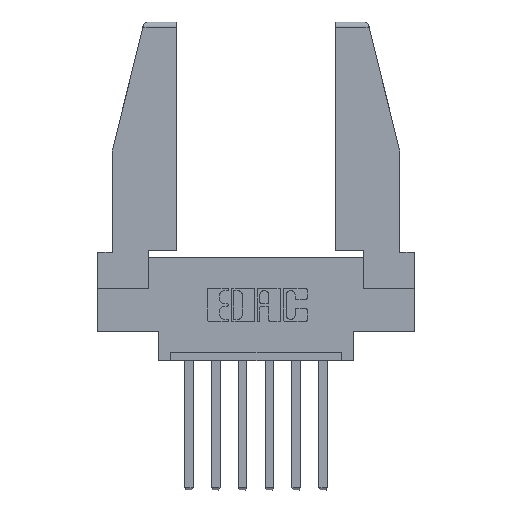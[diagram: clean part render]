
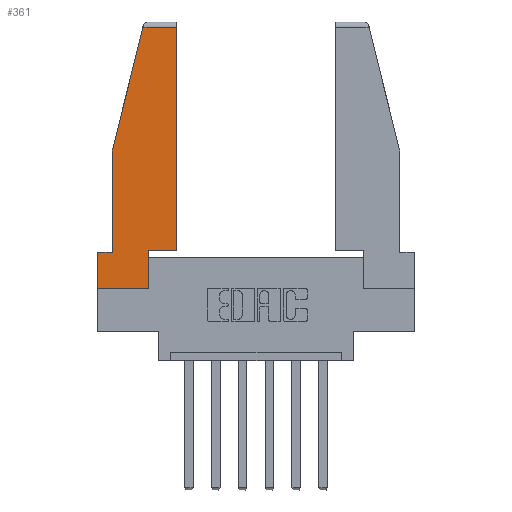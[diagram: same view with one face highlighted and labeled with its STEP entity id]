
A CAD part, top view. The second image highlights one B-rep face of the part: STEP entity #361.
In plain terms, the highlighted planar face has unit normal (0, 0, 1).
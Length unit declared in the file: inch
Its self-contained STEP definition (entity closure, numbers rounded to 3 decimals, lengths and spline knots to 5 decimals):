
#76 = VECTOR ( 'NONE', #7439, 39.37008 ) ;
#149 = VECTOR ( 'NONE', #5746, 39.37008 ) ;
#361 = ADVANCED_FACE ( 'NONE', ( #3894 ), #3486, .T. ) ;
#385 = CARTESIAN_POINT ( 'NONE',  ( 0., 0.21, 0. ) ) ;
#626 = ORIENTED_EDGE ( 'NONE', *, *, #6270, .T. ) ;
#740 = EDGE_CURVE ( 'NONE', #3616, #10870, #2608, .T. ) ;
#2084 = VECTOR ( 'NONE', #3335, 39.37008 ) ;
#2313 = LINE ( 'NONE', #10133, #11498 ) ;
#2318 = ORIENTED_EDGE ( 'NONE', *, *, #4120, .T. ) ;
#2553 = VERTEX_POINT ( 'NONE', #7074 ) ;
#2608 = LINE ( 'NONE', #7267, #2751 ) ;
#2626 = VECTOR ( 'NONE', #10474, 39.37008 ) ;
#2751 = VECTOR ( 'NONE', #9202, 39.37008 ) ;
#3041 = CARTESIAN_POINT ( 'NONE',  ( 0.086, 0.21, 0. ) ) ;
#3116 = ORIENTED_EDGE ( 'NONE', *, *, #9472, .T. ) ;
#3146 = CARTESIAN_POINT ( 'NONE',  ( 0.2636, 1.52, 0. ) ) ;
#3170 = VECTOR ( 'NONE', #8428, 39.37008 ) ;
#3335 = DIRECTION ( 'NONE',  ( 0., -1., 0. ) ) ;
#3486 = PLANE ( 'NONE',  #11102 ) ;
#3616 = VERTEX_POINT ( 'NONE', #3146 ) ;
#3618 = LINE ( 'NONE', #9790, #2626 ) ;
#3780 = LINE ( 'NONE', #10277, #149 ) ;
#3782 = ORIENTED_EDGE ( 'NONE', *, *, #4172, .T. ) ;
#3845 = DIRECTION ( 'NONE',  ( 1., 0., 0. ) ) ;
#3894 = FACE_OUTER_BOUND ( 'NONE', #5212, .T. ) ;
#4120 = EDGE_CURVE ( 'NONE', #10870, #5507, #9185, .T. ) ;
#4172 = EDGE_CURVE ( 'NONE', #7323, #3616, #5680, .T. ) ;
#4372 = DIRECTION ( 'NONE',  ( 1., 0., 0. ) ) ;
#4837 = CARTESIAN_POINT ( 'NONE',  ( 0.086, 0.8, 0. ) ) ;
#5212 = EDGE_LOOP ( 'NONE', ( #7995, #3782, #9319, #2318, #3116, #6295, #626, #8586, #10837 ) ) ;
#5507 = VERTEX_POINT ( 'NONE', #3041 ) ;
#5680 = LINE ( 'NONE', #6605, #3170 ) ;
#5708 = CARTESIAN_POINT ( 'NONE',  ( 0.297, 0.223, 0. ) ) ;
#5746 = DIRECTION ( 'NONE',  ( 0., 1., 0. ) ) ;
#5966 = VECTOR ( 'NONE', #7519, 39.37008 ) ;
#6060 = VECTOR ( 'NONE', #10215, 39.37008 ) ;
#6270 = EDGE_CURVE ( 'NONE', #10476, #2553, #2313, .T. ) ;
#6295 = ORIENTED_EDGE ( 'NONE', *, *, #9051, .T. ) ;
#6425 = EDGE_CURVE ( 'NONE', #9236, #7323, #8443, .T. ) ;
#6564 = EDGE_CURVE ( 'NONE', #10637, #9236, #10944, .T. ) ;
#6605 = CARTESIAN_POINT ( 'NONE',  ( 0., 1.52, 0. ) ) ;
#6821 = CARTESIAN_POINT ( 'NONE',  ( 0.461, 1.52, 0. ) ) ;
#7074 = CARTESIAN_POINT ( 'NONE',  ( 0.297, 0., 0. ) ) ;
#7140 = CARTESIAN_POINT ( 'NONE',  ( 0., 0., 0. ) ) ;
#7267 = CARTESIAN_POINT ( 'NONE',  ( 0.271, 1.55, 0. ) ) ;
#7323 = VERTEX_POINT ( 'NONE', #6821 ) ;
#7439 = DIRECTION ( 'NONE',  ( 1., 0., 0. ) ) ;
#7519 = DIRECTION ( 'NONE',  ( 0., -1., 0. ) ) ;
#7605 = CARTESIAN_POINT ( 'NONE',  ( 0.086, 0.8, 0. ) ) ;
#7822 = LINE ( 'NONE', #10575, #2084 ) ;
#7995 = ORIENTED_EDGE ( 'NONE', *, *, #6425, .T. ) ;
#8428 = DIRECTION ( 'NONE',  ( -1., 0., 0. ) ) ;
#8443 = LINE ( 'NONE', #8508, #6060 ) ;
#8455 = CARTESIAN_POINT ( 'NONE',  ( 0.297, 0.223, 0. ) ) ;
#8507 = CARTESIAN_POINT ( 'NONE',  ( 0., 0., 0. ) ) ;
#8508 = CARTESIAN_POINT ( 'NONE',  ( 0.461, 0.223, 0. ) ) ;
#8586 = ORIENTED_EDGE ( 'NONE', *, *, #8911, .T. ) ;
#8911 = EDGE_CURVE ( 'NONE', #2553, #10637, #3780, .T. ) ;
#8949 = DIRECTION ( 'NONE',  ( 0., 0., 1. ) ) ;
#9021 = CARTESIAN_POINT ( 'NONE',  ( 0.461, 0.223, 0. ) ) ;
#9051 = EDGE_CURVE ( 'NONE', #9625, #10476, #7822, .T. ) ;
#9185 = LINE ( 'NONE', #7605, #5966 ) ;
#9202 = DIRECTION ( 'NONE',  ( -0.239, -0.971, 0. ) ) ;
#9236 = VERTEX_POINT ( 'NONE', #9021 ) ;
#9319 = ORIENTED_EDGE ( 'NONE', *, *, #740, .T. ) ;
#9472 = EDGE_CURVE ( 'NONE', #5507, #9625, #3618, .T. ) ;
#9625 = VERTEX_POINT ( 'NONE', #385 ) ;
#9790 = CARTESIAN_POINT ( 'NONE',  ( 0., 0.21, 0. ) ) ;
#10133 = CARTESIAN_POINT ( 'NONE',  ( 0., 0., 0. ) ) ;
#10215 = DIRECTION ( 'NONE',  ( 0., 1., 0. ) ) ;
#10277 = CARTESIAN_POINT ( 'NONE',  ( 0.297, 0., 0. ) ) ;
#10474 = DIRECTION ( 'NONE',  ( -1., 0., 0. ) ) ;
#10476 = VERTEX_POINT ( 'NONE', #8507 ) ;
#10575 = CARTESIAN_POINT ( 'NONE',  ( 0., 0.21, 0. ) ) ;
#10637 = VERTEX_POINT ( 'NONE', #8455 ) ;
#10837 = ORIENTED_EDGE ( 'NONE', *, *, #6564, .T. ) ;
#10870 = VERTEX_POINT ( 'NONE', #4837 ) ;
#10944 = LINE ( 'NONE', #5708, #76 ) ;
#11102 = AXIS2_PLACEMENT_3D ( 'NONE', #7140, #8949, #4372 ) ;
#11498 = VECTOR ( 'NONE', #3845, 39.37008 ) ;
